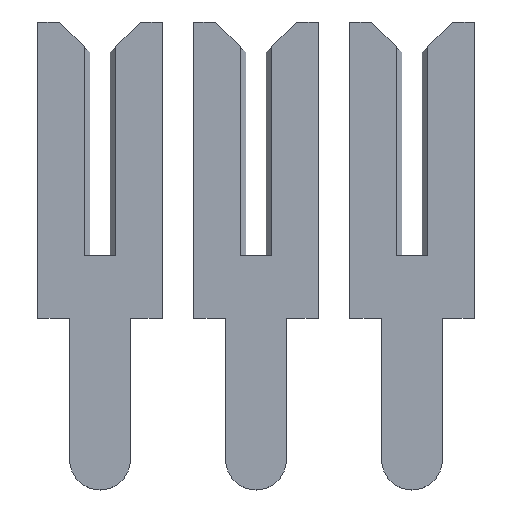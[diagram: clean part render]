
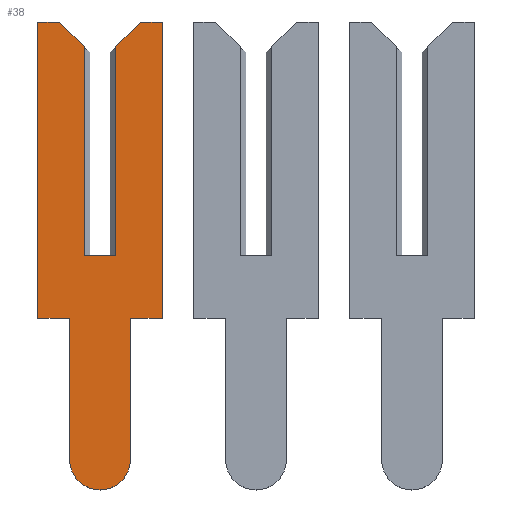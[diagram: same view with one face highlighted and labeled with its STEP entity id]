
A CAD part, top view. The second image highlights one B-rep face of the part: STEP entity #38.
In plain terms, the highlighted face is planar.
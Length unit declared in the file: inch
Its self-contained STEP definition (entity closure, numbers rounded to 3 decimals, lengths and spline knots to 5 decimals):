
#16 = VERTEX_POINT ( 'NONE', #868 ) ;
#27 = CARTESIAN_POINT ( 'NONE',  ( -0.01, -0.1305, -0.01 ) ) ;
#33 = VECTOR ( 'NONE', #867, 39.37008 ) ;
#34 = CARTESIAN_POINT ( 'NONE',  ( -0.01, 0., -0.01 ) ) ;
#38 = ADVANCED_FACE ( 'NONE', ( #852 ), #735, .F. ) ;
#40 = VERTEX_POINT ( 'NONE', #200 ) ;
#41 = CARTESIAN_POINT ( 'NONE',  ( -0.01, -0.1305, 0. ) ) ;
#51 = LINE ( 'NONE', #422, #760 ) ;
#55 = EDGE_CURVE ( 'NONE', #394, #593, #476, .T. ) ;
#70 = ORIENTED_EDGE ( 'NONE', *, *, #888, .F. ) ;
#76 = LINE ( 'NONE', #756, #217 ) ;
#90 = DIRECTION ( 'NONE',  ( 0., -1., 0. ) ) ;
#98 = CARTESIAN_POINT ( 'NONE',  ( -0.01, -0.1305, -0.0195 ) ) ;
#119 = DIRECTION ( 'NONE',  ( 0., 0., -1. ) ) ;
#146 = LINE ( 'NONE', #248, #781 ) ;
#148 = VERTEX_POINT ( 'NONE', #887 ) ;
#149 = ORIENTED_EDGE ( 'NONE', *, *, #698, .F. ) ;
#152 = CARTESIAN_POINT ( 'NONE',  ( -0.01, 0.134, -0.01 ) ) ;
#160 = VECTOR ( 'NONE', #230, 39.37008 ) ;
#161 = CARTESIAN_POINT ( 'NONE',  ( -0.01, -0.04, 0.0195 ) ) ;
#166 = CARTESIAN_POINT ( 'NONE',  ( -0.01, 0.15, -0.026 ) ) ;
#169 = VERTEX_POINT ( 'NONE', #879 ) ;
#171 = LINE ( 'NONE', #331, #522 ) ;
#174 = DIRECTION ( 'NONE',  ( 1., 0., 0. ) ) ;
#175 = EDGE_CURVE ( 'NONE', #16, #206, #51, .T. ) ;
#189 = DIRECTION ( 'NONE',  ( 1., 0., 0. ) ) ;
#191 = DIRECTION ( 'NONE',  ( 0., 0., 1. ) ) ;
#198 = EDGE_CURVE ( 'NONE', #697, #598, #893, .T. ) ;
#200 = CARTESIAN_POINT ( 'NONE',  ( -0.01, -0.04, -0.04 ) ) ;
#206 = VERTEX_POINT ( 'NONE', #810 ) ;
#207 = DIRECTION ( 'NONE',  ( 0., 0., -1. ) ) ;
#208 = ORIENTED_EDGE ( 'NONE', *, *, #299, .F. ) ;
#217 = VECTOR ( 'NONE', #434, 39.37008 ) ;
#230 = DIRECTION ( 'NONE',  ( 0., -0.707, 0.707 ) ) ;
#238 = AXIS2_PLACEMENT_3D ( 'NONE', #397, #174, #720 ) ;
#239 = LINE ( 'NONE', #877, #33 ) ;
#240 = LINE ( 'NONE', #819, #758 ) ;
#248 = CARTESIAN_POINT ( 'NONE',  ( -0.01, 0.15, 0.04 ) ) ;
#256 = EDGE_LOOP ( 'NONE', ( #784, #794, #861, #349, #661, #208, #620, #339, #149, #660, #554, #426, #70, #621 ) ) ;
#257 = EDGE_CURVE ( 'NONE', #169, #40, #240, .T. ) ;
#291 = LINE ( 'NONE', #762, #629 ) ;
#299 = EDGE_CURVE ( 'NONE', #40, #394, #76, .T. ) ;
#312 = LINE ( 'NONE', #561, #160 ) ;
#321 = EDGE_CURVE ( 'NONE', #593, #419, #312, .T. ) ;
#331 = CARTESIAN_POINT ( 'NONE',  ( -0.01, 0.15, 0.026 ) ) ;
#339 = ORIENTED_EDGE ( 'NONE', *, *, #812, .F. ) ;
#349 = ORIENTED_EDGE ( 'NONE', *, *, #321, .F. ) ;
#353 = DIRECTION ( 'NONE',  ( 0., -1., 0. ) ) ;
#372 = DIRECTION ( 'NONE',  ( 0., 0., 1. ) ) ;
#385 = CARTESIAN_POINT ( 'NONE',  ( -0.01, 0., 0.01 ) ) ;
#389 = CARTESIAN_POINT ( 'NONE',  ( -0.01, 0.15, 0.026 ) ) ;
#390 = VECTOR ( 'NONE', #353, 39.37008 ) ;
#391 = LINE ( 'NONE', #558, #830 ) ;
#394 = VERTEX_POINT ( 'NONE', #638 ) ;
#397 = CARTESIAN_POINT ( 'NONE',  ( -0.01, -0.1305, 0. ) ) ;
#399 = DIRECTION ( 'NONE',  ( 0., 0., 1. ) ) ;
#412 = EDGE_CURVE ( 'NONE', #806, #598, #291, .T. ) ;
#419 = VERTEX_POINT ( 'NONE', #152 ) ;
#421 = EDGE_CURVE ( 'NONE', #697, #699, #391, .T. ) ;
#422 = CARTESIAN_POINT ( 'NONE',  ( -0.01, -0.04, 0.04 ) ) ;
#426 = ORIENTED_EDGE ( 'NONE', *, *, #453, .F. ) ;
#434 = DIRECTION ( 'NONE',  ( 0., 1., 0. ) ) ;
#453 = EDGE_CURVE ( 'NONE', #652, #16, #146, .T. ) ;
#460 = VECTOR ( 'NONE', #858, 39.37008 ) ;
#475 = LINE ( 'NONE', #161, #759 ) ;
#476 = LINE ( 'NONE', #791, #630 ) ;
#507 = DIRECTION ( 'NONE',  ( 0., 0.707, 0.707 ) ) ;
#514 = LINE ( 'NONE', #27, #460 ) ;
#522 = VECTOR ( 'NONE', #191, 39.37008 ) ;
#531 = VERTEX_POINT ( 'NONE', #98 ) ;
#549 = CARTESIAN_POINT ( 'NONE',  ( -0.01, 0.15, 0.01 ) ) ;
#554 = ORIENTED_EDGE ( 'NONE', *, *, #175, .F. ) ;
#557 = EDGE_CURVE ( 'NONE', #206, #148, #475, .T. ) ;
#558 = CARTESIAN_POINT ( 'NONE',  ( -0.01, 0.1305, 0.0065 ) ) ;
#561 = CARTESIAN_POINT ( 'NONE',  ( -0.01, 0.1305, -0.0065 ) ) ;
#575 = CARTESIAN_POINT ( 'NONE',  ( -0.01, 0.15, 0.04 ) ) ;
#593 = VERTEX_POINT ( 'NONE', #166 ) ;
#598 = VERTEX_POINT ( 'NONE', #385 ) ;
#620 = ORIENTED_EDGE ( 'NONE', *, *, #257, .F. ) ;
#621 = ORIENTED_EDGE ( 'NONE', *, *, #421, .F. ) ;
#622 = DIRECTION ( 'NONE',  ( 0., 0., -1. ) ) ;
#629 = VECTOR ( 'NONE', #372, 39.37008 ) ;
#630 = VECTOR ( 'NONE', #399, 39.37008 ) ;
#638 = CARTESIAN_POINT ( 'NONE',  ( -0.01, 0.15, -0.04 ) ) ;
#650 = DIRECTION ( 'NONE',  ( 0., -1., 0. ) ) ;
#652 = VERTEX_POINT ( 'NONE', #575 ) ;
#660 = ORIENTED_EDGE ( 'NONE', *, *, #557, .F. ) ;
#661 = ORIENTED_EDGE ( 'NONE', *, *, #55, .F. ) ;
#697 = VERTEX_POINT ( 'NONE', #855 ) ;
#698 = EDGE_CURVE ( 'NONE', #148, #531, #722, .T. ) ;
#699 = VERTEX_POINT ( 'NONE', #389 ) ;
#720 = DIRECTION ( 'NONE',  ( 0., 0., -1. ) ) ;
#722 = CIRCLE ( 'NONE', #238, 0.0195 ) ;
#735 = PLANE ( 'NONE',  #789 ) ;
#756 = CARTESIAN_POINT ( 'NONE',  ( -0.01, 0.15, -0.04 ) ) ;
#758 = VECTOR ( 'NONE', #622, 39.37008 ) ;
#759 = VECTOR ( 'NONE', #90, 39.37008 ) ;
#760 = VECTOR ( 'NONE', #207, 39.37008 ) ;
#761 = EDGE_CURVE ( 'NONE', #419, #806, #514, .T. ) ;
#762 = CARTESIAN_POINT ( 'NONE',  ( -0.01, 0., 0.0065 ) ) ;
#781 = VECTOR ( 'NONE', #650, 39.37008 ) ;
#784 = ORIENTED_EDGE ( 'NONE', *, *, #198, .T. ) ;
#789 = AXIS2_PLACEMENT_3D ( 'NONE', #41, #189, #119 ) ;
#791 = CARTESIAN_POINT ( 'NONE',  ( -0.01, 0.15, -0.026 ) ) ;
#794 = ORIENTED_EDGE ( 'NONE', *, *, #412, .F. ) ;
#806 = VERTEX_POINT ( 'NONE', #34 ) ;
#810 = CARTESIAN_POINT ( 'NONE',  ( -0.01, -0.04, 0.0195 ) ) ;
#812 = EDGE_CURVE ( 'NONE', #531, #169, #239, .T. ) ;
#819 = CARTESIAN_POINT ( 'NONE',  ( -0.01, -0.04, -0.04 ) ) ;
#830 = VECTOR ( 'NONE', #507, 39.37008 ) ;
#852 = FACE_OUTER_BOUND ( 'NONE', #256, .T. ) ;
#855 = CARTESIAN_POINT ( 'NONE',  ( -0.01, 0.134, 0.01 ) ) ;
#858 = DIRECTION ( 'NONE',  ( 0., -1., 0. ) ) ;
#861 = ORIENTED_EDGE ( 'NONE', *, *, #761, .F. ) ;
#867 = DIRECTION ( 'NONE',  ( 0., 1., 0. ) ) ;
#868 = CARTESIAN_POINT ( 'NONE',  ( -0.01, -0.04, 0.04 ) ) ;
#877 = CARTESIAN_POINT ( 'NONE',  ( -0.01, -0.04, -0.0195 ) ) ;
#879 = CARTESIAN_POINT ( 'NONE',  ( -0.01, -0.04, -0.0195 ) ) ;
#887 = CARTESIAN_POINT ( 'NONE',  ( -0.01, -0.1305, 0.0195 ) ) ;
#888 = EDGE_CURVE ( 'NONE', #699, #652, #171, .T. ) ;
#893 = LINE ( 'NONE', #549, #390 ) ;
